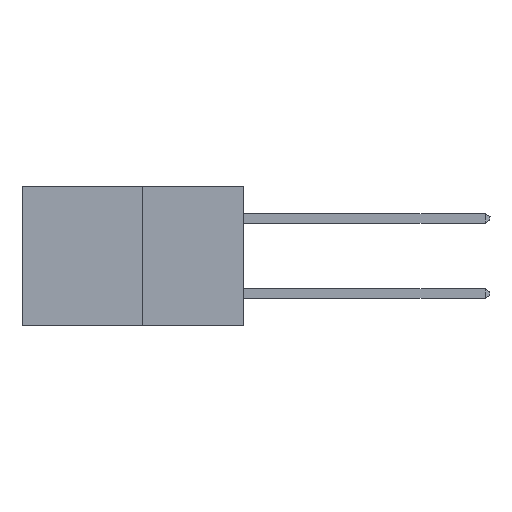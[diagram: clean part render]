
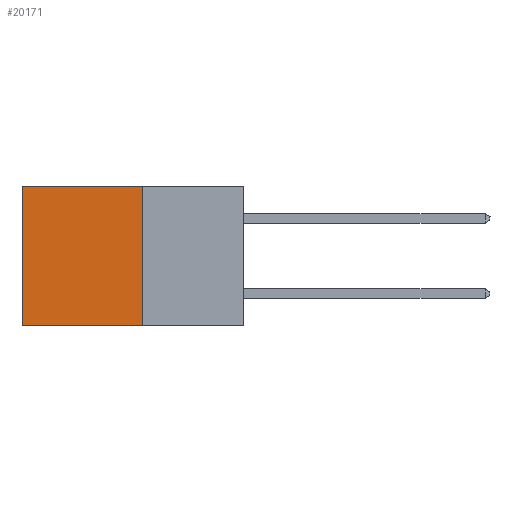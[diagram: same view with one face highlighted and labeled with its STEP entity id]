
A CAD part, left-side view. The second image highlights one B-rep face of the part: STEP entity #20171.
In plain terms, the highlighted planar face has unit normal (-1, 0, 0).
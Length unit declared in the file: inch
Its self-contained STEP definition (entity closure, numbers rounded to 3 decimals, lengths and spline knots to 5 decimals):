
#193 = ORIENTED_EDGE ( 'NONE', *, *, #23074, .F. ) ;
#971 = LINE ( 'NONE', #22744, #22384 ) ;
#1925 = VERTEX_POINT ( 'NONE', #10861 ) ;
#3735 = DIRECTION ( 'NONE',  ( 1., 0., 0. ) ) ;
#4086 = ORIENTED_EDGE ( 'NONE', *, *, #11343, .T. ) ;
#4187 = VERTEX_POINT ( 'NONE', #20642 ) ;
#4994 = CARTESIAN_POINT ( 'NONE',  ( 0.277, 0.27, -0.37 ) ) ;
#5150 = CARTESIAN_POINT ( 'NONE',  ( 0.277, 0.27, 0. ) ) ;
#5868 = EDGE_CURVE ( 'NONE', #24134, #1925, #11786, .T. ) ;
#7105 = DIRECTION ( 'NONE',  ( 0., 0., -1. ) ) ;
#7156 = CARTESIAN_POINT ( 'NONE',  ( 0.277, 0.27, 0. ) ) ;
#7919 = DIRECTION ( 'NONE',  ( 0., 1., 0. ) ) ;
#8112 = VECTOR ( 'NONE', #7105, 39.37008 ) ;
#8779 = LINE ( 'NONE', #17702, #8112 ) ;
#9542 = ORIENTED_EDGE ( 'NONE', *, *, #5868, .T. ) ;
#10861 = CARTESIAN_POINT ( 'NONE',  ( 0.277, 0.59, 0. ) ) ;
#10981 = EDGE_LOOP ( 'NONE', ( #4086, #193, #23181, #9542 ) ) ;
#11343 = EDGE_CURVE ( 'NONE', #1925, #4187, #8779, .T. ) ;
#11786 = LINE ( 'NONE', #7156, #27267 ) ;
#13616 = VECTOR ( 'NONE', #19141, 39.37008 ) ;
#16528 = CARTESIAN_POINT ( 'NONE',  ( 0.277, 0.27, -0.37 ) ) ;
#16980 = CARTESIAN_POINT ( 'NONE',  ( 0.277, 0.27, -0.37 ) ) ;
#17702 = CARTESIAN_POINT ( 'NONE',  ( 0.277, 0.59, -0.37 ) ) ;
#18106 = VERTEX_POINT ( 'NONE', #4994 ) ;
#18664 = DIRECTION ( 'NONE',  ( 0., 0., -1. ) ) ;
#19141 = DIRECTION ( 'NONE',  ( 0., 0., -1. ) ) ;
#20171 = ADVANCED_FACE ( 'NONE', ( #22507 ), #22713, .F. ) ;
#20316 = EDGE_CURVE ( 'NONE', #24134, #18106, #26109, .T. ) ;
#20642 = CARTESIAN_POINT ( 'NONE',  ( 0.277, 0.59, -0.37 ) ) ;
#22384 = VECTOR ( 'NONE', #7919, 39.37008 ) ;
#22507 = FACE_OUTER_BOUND ( 'NONE', #10981, .T. ) ;
#22713 = PLANE ( 'NONE',  #25808 ) ;
#22744 = CARTESIAN_POINT ( 'NONE',  ( 0.277, 0.27, -0.37 ) ) ;
#22947 = DIRECTION ( 'NONE',  ( 0., 1., 0. ) ) ;
#23074 = EDGE_CURVE ( 'NONE', #18106, #4187, #971, .T. ) ;
#23181 = ORIENTED_EDGE ( 'NONE', *, *, #20316, .F. ) ;
#24134 = VERTEX_POINT ( 'NONE', #5150 ) ;
#25808 = AXIS2_PLACEMENT_3D ( 'NONE', #16528, #3735, #18664 ) ;
#26109 = LINE ( 'NONE', #16980, #13616 ) ;
#27267 = VECTOR ( 'NONE', #22947, 39.37008 ) ;
